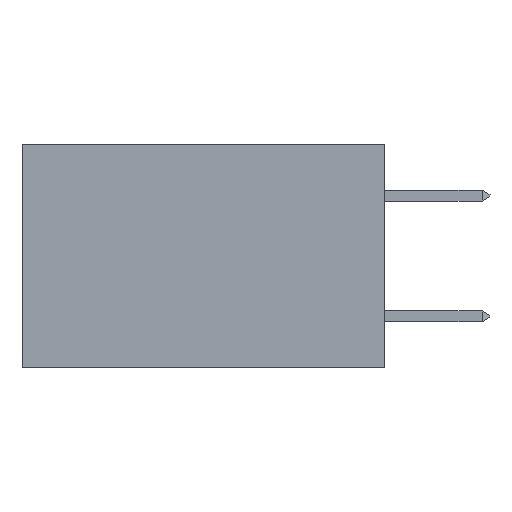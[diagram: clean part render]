
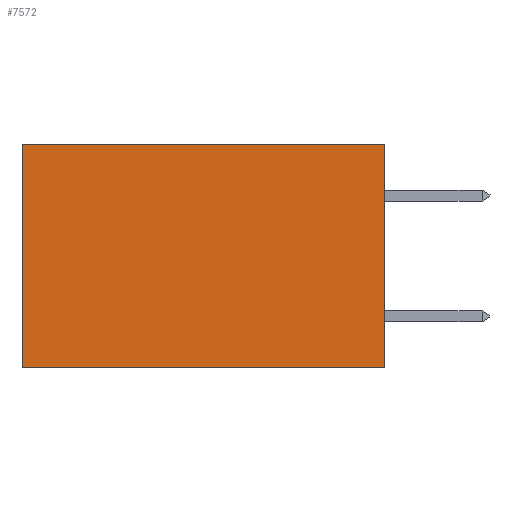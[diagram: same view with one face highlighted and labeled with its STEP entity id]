
A CAD part, left-side view. The second image highlights one B-rep face of the part: STEP entity #7572.
In plain terms, the highlighted planar face has unit normal (-1, 0, 0).
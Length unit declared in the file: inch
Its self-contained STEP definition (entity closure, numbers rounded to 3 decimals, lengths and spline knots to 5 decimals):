
#25 = CARTESIAN_POINT ( 'NONE',  ( 0.2875, 0., 0. ) ) ;
#120 = DIRECTION ( 'NONE',  ( 0., 0., -1. ) ) ;
#549 = CARTESIAN_POINT ( 'NONE',  ( 0.2875, 0.6, -0.37 ) ) ;
#683 = EDGE_LOOP ( 'NONE', ( #3277, #9098, #9107, #5563 ) ) ;
#1046 = EDGE_CURVE ( 'NONE', #1741, #6277, #5099, .T. ) ;
#1741 = VERTEX_POINT ( 'NONE', #11722 ) ;
#2236 = VECTOR ( 'NONE', #2610, 39.37008 ) ;
#2610 = DIRECTION ( 'NONE',  ( 0., 0., -1. ) ) ;
#2719 = LINE ( 'NONE', #13221, #15376 ) ;
#3214 = DIRECTION ( 'NONE',  ( 0., 1., 0. ) ) ;
#3277 = ORIENTED_EDGE ( 'NONE', *, *, #10223, .T. ) ;
#3858 = FACE_OUTER_BOUND ( 'NONE', #683, .T. ) ;
#4351 = EDGE_CURVE ( 'NONE', #15742, #11465, #14385, .T. ) ;
#5099 = LINE ( 'NONE', #9588, #5690 ) ;
#5311 = DIRECTION ( 'NONE',  ( 0., 1., 0. ) ) ;
#5563 = ORIENTED_EDGE ( 'NONE', *, *, #1046, .T. ) ;
#5690 = VECTOR ( 'NONE', #3214, 39.37008 ) ;
#6236 = LINE ( 'NONE', #14754, #2236 ) ;
#6277 = VERTEX_POINT ( 'NONE', #7019 ) ;
#7019 = CARTESIAN_POINT ( 'NONE',  ( 0.2875, 0.6, 0. ) ) ;
#7435 = EDGE_CURVE ( 'NONE', #1741, #15742, #2719, .T. ) ;
#7572 = ADVANCED_FACE ( 'NONE', ( #3858 ), #14697, .F. ) ;
#7868 = VECTOR ( 'NONE', #5311, 39.37008 ) ;
#8945 = CARTESIAN_POINT ( 'NONE',  ( 0.2875, 0., -0.37 ) ) ;
#9098 = ORIENTED_EDGE ( 'NONE', *, *, #4351, .F. ) ;
#9107 = ORIENTED_EDGE ( 'NONE', *, *, #7435, .F. ) ;
#9494 = DIRECTION ( 'NONE',  ( 0., 0., -1. ) ) ;
#9588 = CARTESIAN_POINT ( 'NONE',  ( 0.2875, 0., 0. ) ) ;
#9755 = DIRECTION ( 'NONE',  ( 1., 0., 0. ) ) ;
#10223 = EDGE_CURVE ( 'NONE', #6277, #11465, #6236, .T. ) ;
#11465 = VERTEX_POINT ( 'NONE', #549 ) ;
#11722 = CARTESIAN_POINT ( 'NONE',  ( 0.2875, 0., 0. ) ) ;
#13221 = CARTESIAN_POINT ( 'NONE',  ( 0.2875, 0., 0. ) ) ;
#13320 = CARTESIAN_POINT ( 'NONE',  ( 0.2875, 0., -0.37 ) ) ;
#14385 = LINE ( 'NONE', #8945, #7868 ) ;
#14697 = PLANE ( 'NONE',  #15020 ) ;
#14754 = CARTESIAN_POINT ( 'NONE',  ( 0.2875, 0.6, 0. ) ) ;
#15020 = AXIS2_PLACEMENT_3D ( 'NONE', #25, #9755, #120 ) ;
#15376 = VECTOR ( 'NONE', #9494, 39.37008 ) ;
#15742 = VERTEX_POINT ( 'NONE', #13320 ) ;
